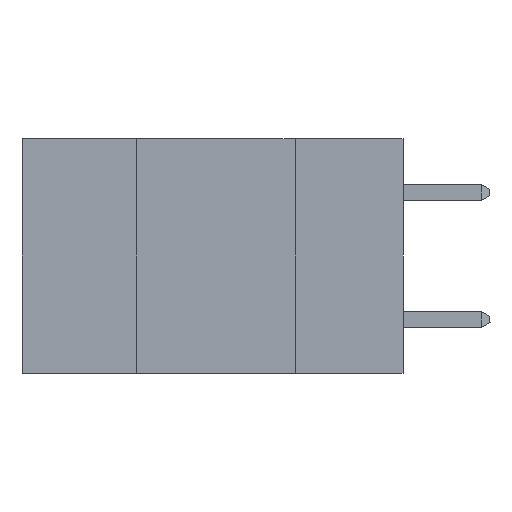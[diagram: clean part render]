
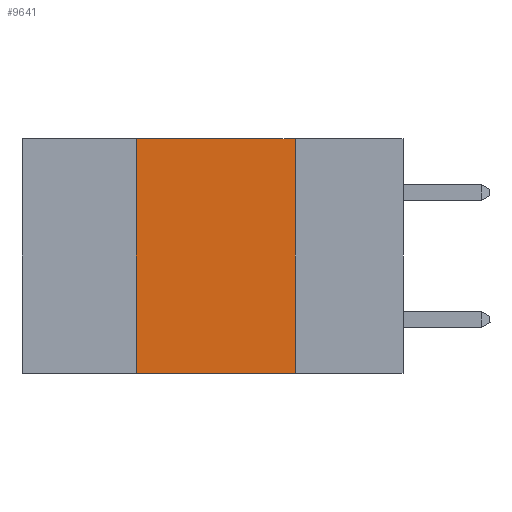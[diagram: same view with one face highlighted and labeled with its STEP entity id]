
A CAD part, left-side view. The second image highlights one B-rep face of the part: STEP entity #9641.
In plain terms, the highlighted planar face has unit normal (-1, 0, 0).
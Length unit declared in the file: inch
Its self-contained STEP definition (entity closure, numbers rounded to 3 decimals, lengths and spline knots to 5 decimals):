
#75 = EDGE_CURVE ( 'NONE', #12790, #20758, #10443, .T. ) ;
#325 = VECTOR ( 'NONE', #23741, 39.37008 ) ;
#373 = ORIENTED_EDGE ( 'NONE', *, *, #11804, .T. ) ;
#1477 = DIRECTION ( 'NONE',  ( 0., 0., -1. ) ) ;
#2916 = CARTESIAN_POINT ( 'NONE',  ( 0., 0.6, -0.37 ) ) ;
#3566 = DIRECTION ( 'NONE',  ( 0., -1., 0. ) ) ;
#4748 = CARTESIAN_POINT ( 'NONE',  ( 0., 0.42, 0. ) ) ;
#4935 = CARTESIAN_POINT ( 'NONE',  ( 0., 0.42, -0.37 ) ) ;
#5313 = CARTESIAN_POINT ( 'NONE',  ( 0., 0.17, 0. ) ) ;
#6072 = ORIENTED_EDGE ( 'NONE', *, *, #20815, .F. ) ;
#7028 = CARTESIAN_POINT ( 'NONE',  ( 0., 0.42, 0. ) ) ;
#7087 = LINE ( 'NONE', #2916, #21648 ) ;
#7553 = LINE ( 'NONE', #23788, #20964 ) ;
#7614 = ORIENTED_EDGE ( 'NONE', *, *, #75, .F. ) ;
#8976 = PLANE ( 'NONE',  #23903 ) ;
#9641 = ADVANCED_FACE ( 'NONE', ( #12411 ), #8976, .F. ) ;
#10443 = LINE ( 'NONE', #5313, #325 ) ;
#11657 = LINE ( 'NONE', #7028, #20685 ) ;
#11804 = EDGE_CURVE ( 'NONE', #14873, #20758, #7087, .T. ) ;
#12411 = FACE_OUTER_BOUND ( 'NONE', #18341, .T. ) ;
#12781 = DIRECTION ( 'NONE',  ( 1., 0., 0. ) ) ;
#12790 = VERTEX_POINT ( 'NONE', #22481 ) ;
#12984 = ORIENTED_EDGE ( 'NONE', *, *, #20167, .F. ) ;
#14873 = VERTEX_POINT ( 'NONE', #4935 ) ;
#15898 = DIRECTION ( 'NONE',  ( 0., -1., 0. ) ) ;
#18341 = EDGE_LOOP ( 'NONE', ( #7614, #6072, #12984, #373 ) ) ;
#20167 = EDGE_CURVE ( 'NONE', #14873, #21245, #11657, .T. ) ;
#20685 = VECTOR ( 'NONE', #21626, 39.37008 ) ;
#20758 = VERTEX_POINT ( 'NONE', #21759 ) ;
#20815 = EDGE_CURVE ( 'NONE', #21245, #12790, #7553, .T. ) ;
#20964 = VECTOR ( 'NONE', #3566, 39.37008 ) ;
#21245 = VERTEX_POINT ( 'NONE', #4748 ) ;
#21626 = DIRECTION ( 'NONE',  ( 0., 0., 1. ) ) ;
#21648 = VECTOR ( 'NONE', #15898, 39.37008 ) ;
#21759 = CARTESIAN_POINT ( 'NONE',  ( 0., 0.17, -0.37 ) ) ;
#22481 = CARTESIAN_POINT ( 'NONE',  ( 0., 0.17, 0. ) ) ;
#23663 = CARTESIAN_POINT ( 'NONE',  ( 0., 0.6, 0. ) ) ;
#23741 = DIRECTION ( 'NONE',  ( 0., 0., -1. ) ) ;
#23788 = CARTESIAN_POINT ( 'NONE',  ( 0., 0.6, 0. ) ) ;
#23903 = AXIS2_PLACEMENT_3D ( 'NONE', #23663, #12781, #1477 ) ;
